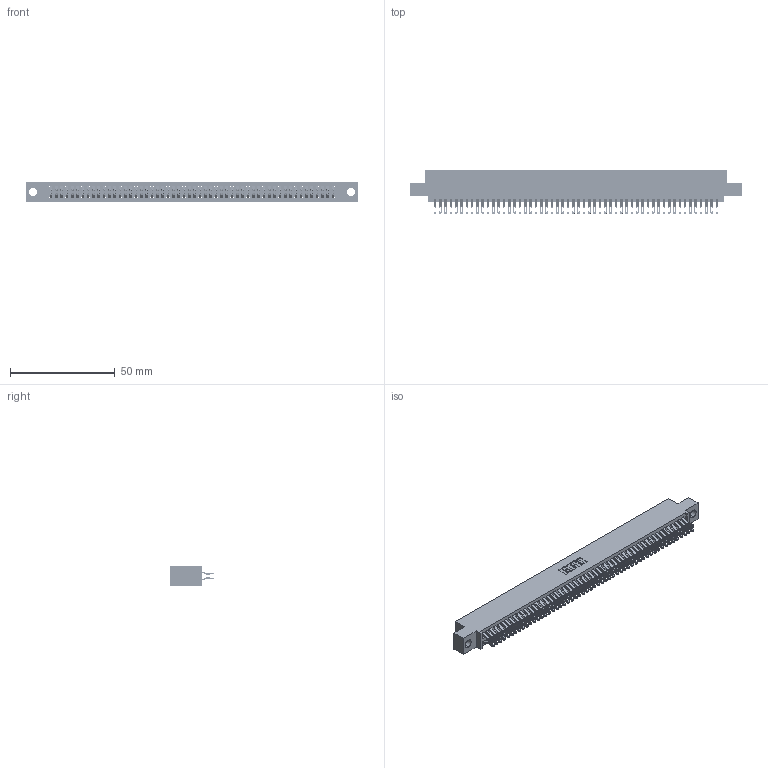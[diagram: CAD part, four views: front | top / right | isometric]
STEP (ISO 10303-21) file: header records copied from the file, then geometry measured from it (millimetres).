
FILE_DESCRIPTION (( 'STEP AP203' ), '1' );
FILE_NAME ('395-108-555-504.STEP', '2018-11-30T23:11:49', ( '' ), ( '' ), 'SwSTEP 2.0', 'SolidWorks 2016', '' );
FILE_SCHEMA (( 'CONFIG_CONTROL_DESIGN' ));
Length unit declared in the file: inch
Products named in the file (3): 395-108-555-504; 345-292-001_555 Tail; 345 Part_0.110 Offset - 0.156 Dia-TH
Assembly tree (109 placements, depth 2):
  395-108-555-504
    345 Part_0.110 Offset - 0.156 Dia-TH
    345-292-001_555 Tail  x108
Bounding box: 158.37 x 21.13 x 9.4 mm (x, y, z)
Volume: 15647.6 mm3; surface area: 24359.7 mm2
Topology: 109 solids, 109 shells, 6178 faces, 19469 edges, 12978 vertices
Faces by surface type: plane 3432, cylinder 2746
Entity records: 41215 total; most frequent: CARTESIAN_POINT 6934, ORIENTED_EDGE 6838, DIRECTION 6067, EDGE_CURVE 3419, VECTOR 3051, LINE 3051, VERTEX_POINT 2278, AXIS2_PLACEMENT_3D 1508
